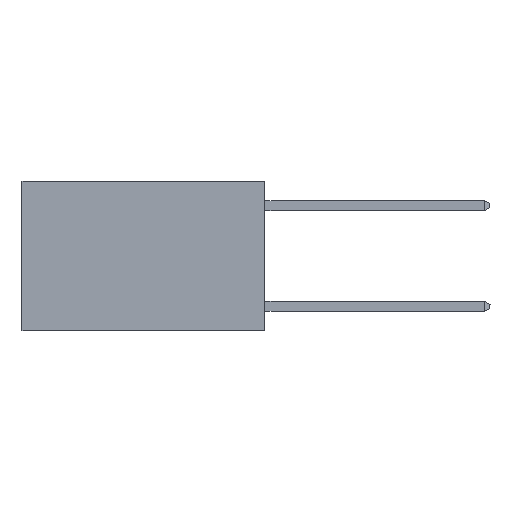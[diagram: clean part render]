
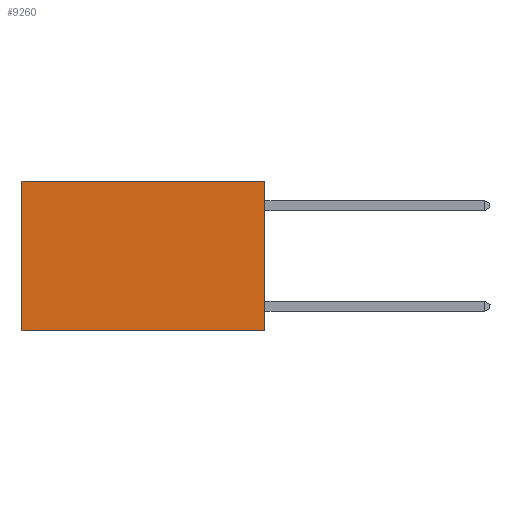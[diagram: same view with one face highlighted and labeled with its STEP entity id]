
A CAD part, left-side view. The second image highlights one B-rep face of the part: STEP entity #9260.
In plain terms, the highlighted planar face has unit normal (-1, 0, 0).
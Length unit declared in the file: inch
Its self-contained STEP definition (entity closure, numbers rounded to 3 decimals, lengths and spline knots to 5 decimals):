
#402 = VECTOR ( 'NONE', #9740, 39.37008 ) ;
#535 = VECTOR ( 'NONE', #9529, 39.37008 ) ;
#568 = ORIENTED_EDGE ( 'NONE', *, *, #9197, .T. ) ;
#688 = VERTEX_POINT ( 'NONE', #3758 ) ;
#727 = DIRECTION ( 'NONE',  ( 0., 0., -1. ) ) ;
#922 = CARTESIAN_POINT ( 'NONE',  ( 0.2625, 0., -0.37 ) ) ;
#923 = CARTESIAN_POINT ( 'NONE',  ( 0.2625, 0.6, -0.37 ) ) ;
#1696 = DIRECTION ( 'NONE',  ( 0., 0., -1. ) ) ;
#1923 = LINE ( 'NONE', #4428, #8923 ) ;
#2029 = FACE_OUTER_BOUND ( 'NONE', #7715, .T. ) ;
#2805 = ORIENTED_EDGE ( 'NONE', *, *, #10531, .T. ) ;
#2848 = VERTEX_POINT ( 'NONE', #922 ) ;
#3405 = CARTESIAN_POINT ( 'NONE',  ( 0.2625, 0., 0. ) ) ;
#3758 = CARTESIAN_POINT ( 'NONE',  ( 0.2625, 0., 0. ) ) ;
#4189 = VERTEX_POINT ( 'NONE', #923 ) ;
#4299 = LINE ( 'NONE', #6092, #10800 ) ;
#4428 = CARTESIAN_POINT ( 'NONE',  ( 0.2625, 0., 0. ) ) ;
#4759 = CARTESIAN_POINT ( 'NONE',  ( 0.2625, 0.6, 0. ) ) ;
#5246 = DIRECTION ( 'NONE',  ( 0., 1., 0. ) ) ;
#5953 = AXIS2_PLACEMENT_3D ( 'NONE', #8971, #6192, #727 ) ;
#6092 = CARTESIAN_POINT ( 'NONE',  ( 0.2625, 0., -0.37 ) ) ;
#6192 = DIRECTION ( 'NONE',  ( 1., 0., 0. ) ) ;
#6678 = EDGE_CURVE ( 'NONE', #2848, #4189, #4299, .T. ) ;
#7715 = EDGE_LOOP ( 'NONE', ( #2805, #9395, #10600, #568 ) ) ;
#8026 = LINE ( 'NONE', #3405, #402 ) ;
#8262 = EDGE_CURVE ( 'NONE', #688, #2848, #1923, .T. ) ;
#8923 = VECTOR ( 'NONE', #1696, 39.37008 ) ;
#8971 = CARTESIAN_POINT ( 'NONE',  ( 0.2625, 0., 0. ) ) ;
#8974 = VERTEX_POINT ( 'NONE', #4759 ) ;
#9197 = EDGE_CURVE ( 'NONE', #688, #8974, #8026, .T. ) ;
#9260 = ADVANCED_FACE ( 'NONE', ( #2029 ), #10646, .F. ) ;
#9395 = ORIENTED_EDGE ( 'NONE', *, *, #6678, .F. ) ;
#9447 = LINE ( 'NONE', #11135, #535 ) ;
#9529 = DIRECTION ( 'NONE',  ( 0., 0., -1. ) ) ;
#9740 = DIRECTION ( 'NONE',  ( 0., 1., 0. ) ) ;
#10531 = EDGE_CURVE ( 'NONE', #8974, #4189, #9447, .T. ) ;
#10600 = ORIENTED_EDGE ( 'NONE', *, *, #8262, .F. ) ;
#10646 = PLANE ( 'NONE',  #5953 ) ;
#10800 = VECTOR ( 'NONE', #5246, 39.37008 ) ;
#11135 = CARTESIAN_POINT ( 'NONE',  ( 0.2625, 0.6, 0. ) ) ;
